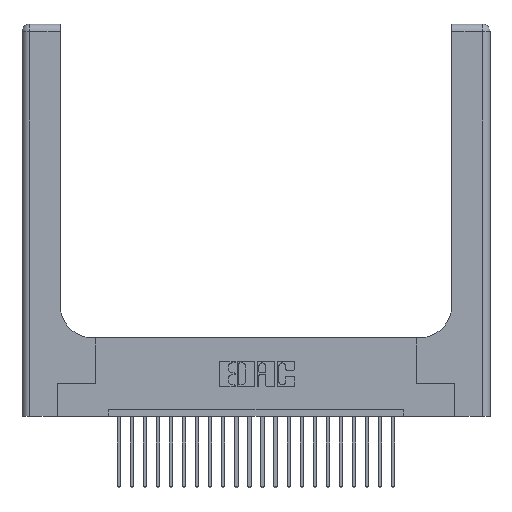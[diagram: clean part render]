
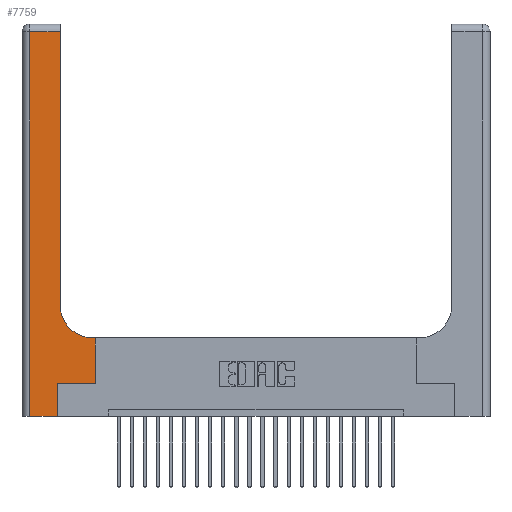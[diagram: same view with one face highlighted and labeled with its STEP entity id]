
A CAD part, top view. The second image highlights one B-rep face of the part: STEP entity #7759.
In plain terms, the highlighted planar face has unit normal (0, 0, 1).
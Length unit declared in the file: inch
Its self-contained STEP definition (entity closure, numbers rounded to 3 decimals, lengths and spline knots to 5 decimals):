
#377 = LINE ( 'NONE', #6228, #19308 ) ;
#381 = LINE ( 'NONE', #15800, #13646 ) ;
#394 = CARTESIAN_POINT ( 'NONE',  ( 0.269, 0., 0.37 ) ) ;
#1248 = CARTESIAN_POINT ( 'NONE',  ( 0.06, 3., 0.37 ) ) ;
#1308 = ORIENTED_EDGE ( 'NONE', *, *, #7983, .T. ) ;
#1516 = ORIENTED_EDGE ( 'NONE', *, *, #10507, .T. ) ;
#1826 = AXIS2_PLACEMENT_3D ( 'NONE', #7676, #6044, #11659 ) ;
#2475 = DIRECTION ( 'NONE',  ( 0., 1., 0. ) ) ;
#2942 = EDGE_CURVE ( 'NONE', #19398, #14328, #19081, .T. ) ;
#3886 = EDGE_CURVE ( 'NONE', #6180, #14687, #11872, .T. ) ;
#4057 = EDGE_CURVE ( 'NONE', #23098, #6180, #377, .T. ) ;
#4254 = DIRECTION ( 'NONE',  ( 0., 1., 0. ) ) ;
#5260 = CARTESIAN_POINT ( 'NONE',  ( 0.5415, 0.6, 0.37 ) ) ;
#5595 = EDGE_CURVE ( 'NONE', #23549, #23098, #21448, .T. ) ;
#6044 = DIRECTION ( 'NONE',  ( 0., 0., -1. ) ) ;
#6180 = VERTEX_POINT ( 'NONE', #11462 ) ;
#6228 = CARTESIAN_POINT ( 'NONE',  ( 0., 2.94, 0.37 ) ) ;
#6638 = ORIENTED_EDGE ( 'NONE', *, *, #16754, .T. ) ;
#7676 = CARTESIAN_POINT ( 'NONE',  ( 0., 3., 0.37 ) ) ;
#7759 = ADVANCED_FACE ( 'NONE', ( #16357 ), #22903, .F. ) ;
#7983 = EDGE_CURVE ( 'NONE', #16221, #19398, #381, .T. ) ;
#8068 = VERTEX_POINT ( 'NONE', #16229 ) ;
#8208 = LINE ( 'NONE', #12800, #11440 ) ;
#8260 = AXIS2_PLACEMENT_3D ( 'NONE', #23907, #18253, #19821 ) ;
#8715 = EDGE_LOOP ( 'NONE', ( #14389, #23351, #11866, #1516, #11281, #9635, #1308, #20443, #6638 ) ) ;
#8940 = DIRECTION ( 'NONE',  ( 1., 0., 0. ) ) ;
#9459 = DIRECTION ( 'NONE',  ( 0., 1., 0. ) ) ;
#9604 = CARTESIAN_POINT ( 'NONE',  ( 0.5585, 0.6, 0.37 ) ) ;
#9635 = ORIENTED_EDGE ( 'NONE', *, *, #9965, .T. ) ;
#9944 = CARTESIAN_POINT ( 'NONE',  ( 0.2915, 0.85, 0.37 ) ) ;
#9965 = EDGE_CURVE ( 'NONE', #19125, #16221, #18917, .T. ) ;
#10507 = EDGE_CURVE ( 'NONE', #14687, #8068, #8208, .T. ) ;
#10695 = EDGE_CURVE ( 'NONE', #8068, #19125, #18594, .T. ) ;
#11281 = ORIENTED_EDGE ( 'NONE', *, *, #10695, .T. ) ;
#11440 = VECTOR ( 'NONE', #24288, 39.37008 ) ;
#11462 = CARTESIAN_POINT ( 'NONE',  ( 0.06, 2.94, 0.37 ) ) ;
#11598 = VECTOR ( 'NONE', #13843, 39.37008 ) ;
#11659 = DIRECTION ( 'NONE',  ( -1., 0., 0. ) ) ;
#11866 = ORIENTED_EDGE ( 'NONE', *, *, #3886, .T. ) ;
#11872 = LINE ( 'NONE', #1248, #11598 ) ;
#11900 = CARTESIAN_POINT ( 'NONE',  ( 0.06, 0., 0.37 ) ) ;
#12800 = CARTESIAN_POINT ( 'NONE',  ( 0., 0., 0.37 ) ) ;
#13593 = CARTESIAN_POINT ( 'NONE',  ( 0.5585, 0.25, 0.37 ) ) ;
#13646 = VECTOR ( 'NONE', #4254, 39.37008 ) ;
#13732 = CARTESIAN_POINT ( 'NONE',  ( 0.2915, 3., 0.37 ) ) ;
#13843 = DIRECTION ( 'NONE',  ( 0., -1., 0. ) ) ;
#14328 = VERTEX_POINT ( 'NONE', #5260 ) ;
#14389 = ORIENTED_EDGE ( 'NONE', *, *, #5595, .T. ) ;
#14687 = VERTEX_POINT ( 'NONE', #11900 ) ;
#14934 = CARTESIAN_POINT ( 'NONE',  ( 0.269, 0.25, 0.37 ) ) ;
#14997 = CIRCLE ( 'NONE', #8260, 0.25 ) ;
#15800 = CARTESIAN_POINT ( 'NONE',  ( 0.5585, 0.25, 0.37 ) ) ;
#16221 = VERTEX_POINT ( 'NONE', #13593 ) ;
#16229 = CARTESIAN_POINT ( 'NONE',  ( 0.269, 0., 0.37 ) ) ;
#16357 = FACE_OUTER_BOUND ( 'NONE', #8715, .T. ) ;
#16754 = EDGE_CURVE ( 'NONE', #14328, #23549, #14997, .T. ) ;
#18253 = DIRECTION ( 'NONE',  ( 0., 0., -1. ) ) ;
#18594 = LINE ( 'NONE', #394, #19471 ) ;
#18917 = LINE ( 'NONE', #24054, #23310 ) ;
#19081 = LINE ( 'NONE', #20575, #24344 ) ;
#19125 = VERTEX_POINT ( 'NONE', #14934 ) ;
#19153 = DIRECTION ( 'NONE',  ( -1., 0., 0. ) ) ;
#19308 = VECTOR ( 'NONE', #19153, 39.37008 ) ;
#19398 = VERTEX_POINT ( 'NONE', #9604 ) ;
#19471 = VECTOR ( 'NONE', #9459, 39.37008 ) ;
#19762 = CARTESIAN_POINT ( 'NONE',  ( 0.2915, 2.94, 0.37 ) ) ;
#19821 = DIRECTION ( 'NONE',  ( 1., 0., 0. ) ) ;
#20292 = DIRECTION ( 'NONE',  ( -1., 0., 0. ) ) ;
#20443 = ORIENTED_EDGE ( 'NONE', *, *, #2942, .T. ) ;
#20575 = CARTESIAN_POINT ( 'NONE',  ( 0.2915, 0.6, 0.37 ) ) ;
#21166 = VECTOR ( 'NONE', #2475, 39.37008 ) ;
#21448 = LINE ( 'NONE', #13732, #21166 ) ;
#22903 = PLANE ( 'NONE',  #1826 ) ;
#23098 = VERTEX_POINT ( 'NONE', #19762 ) ;
#23310 = VECTOR ( 'NONE', #8940, 39.37008 ) ;
#23351 = ORIENTED_EDGE ( 'NONE', *, *, #4057, .T. ) ;
#23549 = VERTEX_POINT ( 'NONE', #9944 ) ;
#23907 = CARTESIAN_POINT ( 'NONE',  ( 0.5415, 0.85, 0.37 ) ) ;
#24054 = CARTESIAN_POINT ( 'NONE',  ( 0.269, 0.25, 0.37 ) ) ;
#24288 = DIRECTION ( 'NONE',  ( 1., 0., 0. ) ) ;
#24344 = VECTOR ( 'NONE', #20292, 39.37008 ) ;
